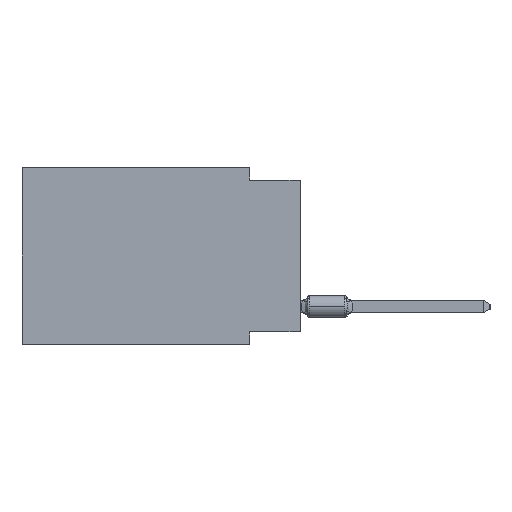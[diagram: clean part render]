
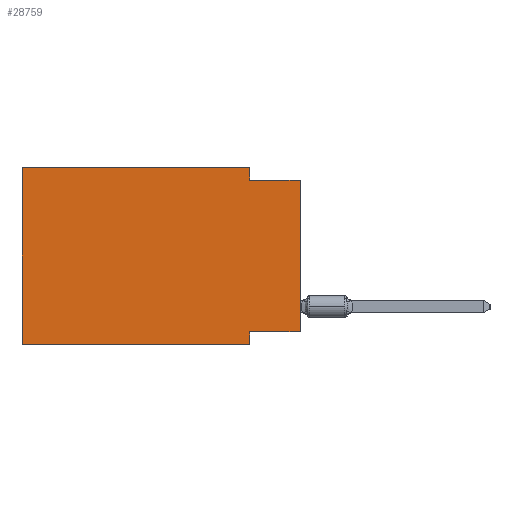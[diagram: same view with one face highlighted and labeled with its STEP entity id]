
A CAD part, left-side view. The second image highlights one B-rep face of the part: STEP entity #28759.
In plain terms, the highlighted planar face has unit normal (-1, 0, 0).
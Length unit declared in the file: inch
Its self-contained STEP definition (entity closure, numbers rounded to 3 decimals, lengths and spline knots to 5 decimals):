
#2066 = LINE ( 'NONE', #2605, #23877 ) ;
#2440 = VERTEX_POINT ( 'NONE', #94368 ) ;
#2605 = CARTESIAN_POINT ( 'NONE',  ( 0., 0., -0.325 ) ) ;
#4743 = CARTESIAN_POINT ( 'NONE',  ( 0., 0., -0.025 ) ) ;
#7487 = ORIENTED_EDGE ( 'NONE', *, *, #20199, .F. ) ;
#8496 = DIRECTION ( 'NONE',  ( 0., 0., 1. ) ) ;
#11154 = CARTESIAN_POINT ( 'NONE',  ( 0., 0.55, -0.35 ) ) ;
#16401 = DIRECTION ( 'NONE',  ( 0., 0., -1. ) ) ;
#17103 = EDGE_CURVE ( 'NONE', #90305, #2440, #93002, .T. ) ;
#18547 = VECTOR ( 'NONE', #105498, 39.37008 ) ;
#19648 = EDGE_CURVE ( 'NONE', #65899, #23010, #36236, .T. ) ;
#20199 = EDGE_CURVE ( 'NONE', #89884, #2440, #72916, .T. ) ;
#20360 = CARTESIAN_POINT ( 'NONE',  ( 0., 0.1, -0.325 ) ) ;
#21737 = CARTESIAN_POINT ( 'NONE',  ( 0., 0., -0.025 ) ) ;
#22097 = VECTOR ( 'NONE', #105345, 39.37008 ) ;
#23010 = VERTEX_POINT ( 'NONE', #49777 ) ;
#23689 = LINE ( 'NONE', #4743, #18547 ) ;
#23877 = VECTOR ( 'NONE', #59536, 39.37008 ) ;
#26388 = ORIENTED_EDGE ( 'NONE', *, *, #19648, .F. ) ;
#27432 = CARTESIAN_POINT ( 'NONE',  ( 0., 0.55, 0. ) ) ;
#27503 = ORIENTED_EDGE ( 'NONE', *, *, #48198, .F. ) ;
#28759 = ADVANCED_FACE ( 'NONE', ( #32110 ), #49981, .F. ) ;
#30138 = CARTESIAN_POINT ( 'NONE',  ( 0., 0.1, -0.35 ) ) ;
#30884 = VERTEX_POINT ( 'NONE', #62523 ) ;
#31654 = LINE ( 'NONE', #72319, #22097 ) ;
#32110 = FACE_OUTER_BOUND ( 'NONE', #95122, .T. ) ;
#33037 = ORIENTED_EDGE ( 'NONE', *, *, #17103, .T. ) ;
#33169 = CARTESIAN_POINT ( 'NONE',  ( 0., 0.55, 0. ) ) ;
#34730 = VERTEX_POINT ( 'NONE', #21737 ) ;
#35184 = CARTESIAN_POINT ( 'NONE',  ( 0., 0.55, 0. ) ) ;
#36073 = DIRECTION ( 'NONE',  ( 0., -1., 0. ) ) ;
#36236 = LINE ( 'NONE', #53042, #68196 ) ;
#36972 = ORIENTED_EDGE ( 'NONE', *, *, #49877, .F. ) ;
#48198 = EDGE_CURVE ( 'NONE', #30884, #89884, #2066, .T. ) ;
#48911 = DIRECTION ( 'NONE',  ( 1., 0., 0. ) ) ;
#49777 = CARTESIAN_POINT ( 'NONE',  ( 0., 0.1, 0. ) ) ;
#49877 = EDGE_CURVE ( 'NONE', #90305, #65899, #101676, .T. ) ;
#49981 = PLANE ( 'NONE',  #64395 ) ;
#51772 = VECTOR ( 'NONE', #85954, 39.37008 ) ;
#53042 = CARTESIAN_POINT ( 'NONE',  ( 0., 0.55, 0. ) ) ;
#58859 = LINE ( 'NONE', #91921, #61797 ) ;
#59536 = DIRECTION ( 'NONE',  ( 0., 1., 0. ) ) ;
#61797 = VECTOR ( 'NONE', #8496, 39.37008 ) ;
#62523 = CARTESIAN_POINT ( 'NONE',  ( 0., 0., -0.325 ) ) ;
#64395 = AXIS2_PLACEMENT_3D ( 'NONE', #33169, #48911, #16401 ) ;
#65899 = VERTEX_POINT ( 'NONE', #35184 ) ;
#67937 = CARTESIAN_POINT ( 'NONE',  ( 0., 0.55, -0.35 ) ) ;
#68196 = VECTOR ( 'NONE', #87718, 39.37008 ) ;
#72319 = CARTESIAN_POINT ( 'NONE',  ( 0., 0.1, 0. ) ) ;
#72916 = LINE ( 'NONE', #30138, #106319 ) ;
#76599 = EDGE_CURVE ( 'NONE', #103821, #34730, #23689, .T. ) ;
#76690 = EDGE_CURVE ( 'NONE', #30884, #34730, #58859, .T. ) ;
#80170 = ORIENTED_EDGE ( 'NONE', *, *, #76599, .F. ) ;
#81069 = DIRECTION ( 'NONE',  ( 0., 0., -1. ) ) ;
#82936 = ORIENTED_EDGE ( 'NONE', *, *, #76690, .T. ) ;
#84762 = ORIENTED_EDGE ( 'NONE', *, *, #104786, .F. ) ;
#85954 = DIRECTION ( 'NONE',  ( 0., 0., 1. ) ) ;
#87718 = DIRECTION ( 'NONE',  ( 0., -1., 0. ) ) ;
#89884 = VERTEX_POINT ( 'NONE', #20360 ) ;
#90305 = VERTEX_POINT ( 'NONE', #67937 ) ;
#91921 = CARTESIAN_POINT ( 'NONE',  ( 0., 0., 0. ) ) ;
#92689 = CARTESIAN_POINT ( 'NONE',  ( 0., 0.1, -0.025 ) ) ;
#93002 = LINE ( 'NONE', #11154, #95501 ) ;
#94368 = CARTESIAN_POINT ( 'NONE',  ( 0., 0.1, -0.35 ) ) ;
#95122 = EDGE_LOOP ( 'NONE', ( #82936, #80170, #84762, #26388, #36972, #33037, #7487, #27503 ) ) ;
#95501 = VECTOR ( 'NONE', #36073, 39.37008 ) ;
#101676 = LINE ( 'NONE', #27432, #51772 ) ;
#103821 = VERTEX_POINT ( 'NONE', #92689 ) ;
#104786 = EDGE_CURVE ( 'NONE', #23010, #103821, #31654, .T. ) ;
#105345 = DIRECTION ( 'NONE',  ( 0., 0., -1. ) ) ;
#105498 = DIRECTION ( 'NONE',  ( 0., -1., 0. ) ) ;
#106319 = VECTOR ( 'NONE', #81069, 39.37008 ) ;
